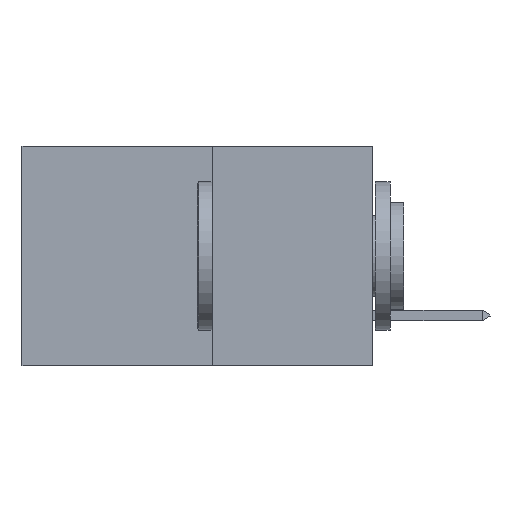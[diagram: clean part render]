
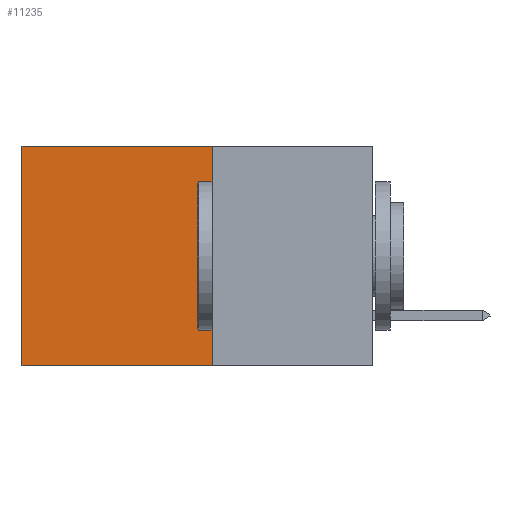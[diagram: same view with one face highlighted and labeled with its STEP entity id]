
A CAD part, left-side view. The second image highlights one B-rep face of the part: STEP entity #11235.
In plain terms, the highlighted planar face has unit normal (-1, 0, 0).
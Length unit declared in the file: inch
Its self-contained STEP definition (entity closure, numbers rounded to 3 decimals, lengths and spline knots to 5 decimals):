
#712 = EDGE_CURVE ( 'NONE', #9542, #8505, #10989, .T. ) ;
#1221 = ORIENTED_EDGE ( 'NONE', *, *, #6392, .T. ) ;
#1648 = ORIENTED_EDGE ( 'NONE', *, *, #712, .F. ) ;
#1885 = CARTESIAN_POINT ( 'NONE',  ( 0.277, 0.27, -0.37 ) ) ;
#2052 = AXIS2_PLACEMENT_3D ( 'NONE', #4841, #11907, #5852 ) ;
#2099 = CARTESIAN_POINT ( 'NONE',  ( 0.277, 0.27, 0. ) ) ;
#2706 = VECTOR ( 'NONE', #12006, 39.37008 ) ;
#2872 = VECTOR ( 'NONE', #12297, 39.37008 ) ;
#2984 = VERTEX_POINT ( 'NONE', #3328 ) ;
#3328 = CARTESIAN_POINT ( 'NONE',  ( 0.277, 0.59, 0. ) ) ;
#3662 = ORIENTED_EDGE ( 'NONE', *, *, #10806, .F. ) ;
#3890 = VECTOR ( 'NONE', #11132, 39.37008 ) ;
#4081 = CARTESIAN_POINT ( 'NONE',  ( 0.277, 0.27, -0.37 ) ) ;
#4513 = VECTOR ( 'NONE', #7764, 39.37008 ) ;
#4841 = CARTESIAN_POINT ( 'NONE',  ( 0.277, 0.27, -0.37 ) ) ;
#5045 = EDGE_LOOP ( 'NONE', ( #6289, #3662, #1648, #1221 ) ) ;
#5262 = VERTEX_POINT ( 'NONE', #8141 ) ;
#5852 = DIRECTION ( 'NONE',  ( 0., 0., -1. ) ) ;
#6289 = ORIENTED_EDGE ( 'NONE', *, *, #6944, .T. ) ;
#6392 = EDGE_CURVE ( 'NONE', #9542, #2984, #8183, .T. ) ;
#6646 = LINE ( 'NONE', #1885, #3890 ) ;
#6944 = EDGE_CURVE ( 'NONE', #2984, #5262, #7258, .T. ) ;
#7258 = LINE ( 'NONE', #7529, #4513 ) ;
#7529 = CARTESIAN_POINT ( 'NONE',  ( 0.277, 0.59, -0.37 ) ) ;
#7764 = DIRECTION ( 'NONE',  ( 0., 0., -1. ) ) ;
#8141 = CARTESIAN_POINT ( 'NONE',  ( 0.277, 0.59, -0.37 ) ) ;
#8183 = LINE ( 'NONE', #2099, #2706 ) ;
#8505 = VERTEX_POINT ( 'NONE', #4081 ) ;
#8873 = FACE_OUTER_BOUND ( 'NONE', #5045, .T. ) ;
#9510 = CARTESIAN_POINT ( 'NONE',  ( 0.277, 0.27, 0. ) ) ;
#9542 = VERTEX_POINT ( 'NONE', #9510 ) ;
#10806 = EDGE_CURVE ( 'NONE', #8505, #5262, #6646, .T. ) ;
#10926 = PLANE ( 'NONE',  #2052 ) ;
#10989 = LINE ( 'NONE', #11289, #2872 ) ;
#11132 = DIRECTION ( 'NONE',  ( 0., 1., 0. ) ) ;
#11235 = ADVANCED_FACE ( 'NONE', ( #8873 ), #10926, .F. ) ;
#11289 = CARTESIAN_POINT ( 'NONE',  ( 0.277, 0.27, -0.37 ) ) ;
#11907 = DIRECTION ( 'NONE',  ( 1., 0., 0. ) ) ;
#12006 = DIRECTION ( 'NONE',  ( 0., 1., 0. ) ) ;
#12297 = DIRECTION ( 'NONE',  ( 0., 0., -1. ) ) ;
